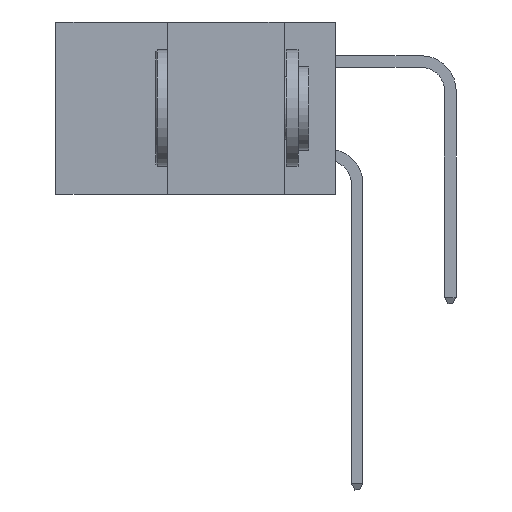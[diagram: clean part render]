
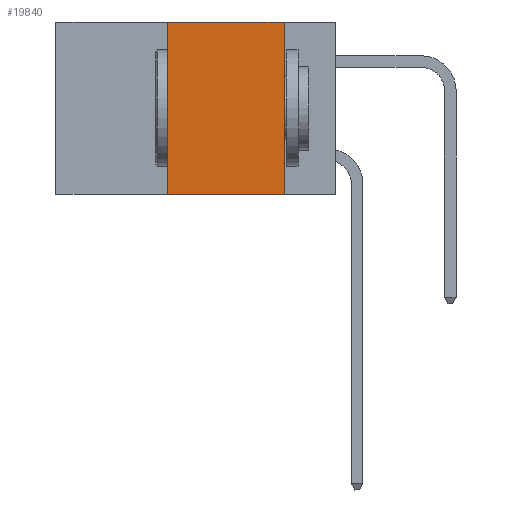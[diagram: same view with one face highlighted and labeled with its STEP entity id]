
A CAD part, left-side view. The second image highlights one B-rep face of the part: STEP entity #19840.
In plain terms, the highlighted planar face has unit normal (-1, 0, 0).
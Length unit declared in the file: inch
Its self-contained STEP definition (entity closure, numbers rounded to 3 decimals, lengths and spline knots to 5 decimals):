
#1787 = ORIENTED_EDGE ( 'NONE', *, *, #14523, .F. ) ;
#3164 = FACE_OUTER_BOUND ( 'NONE', #8803, .T. ) ;
#3603 = CARTESIAN_POINT ( 'NONE',  ( 0., 0.11, -0.37 ) ) ;
#3821 = VECTOR ( 'NONE', #36812, 39.37008 ) ;
#5599 = VECTOR ( 'NONE', #29644, 39.37008 ) ;
#8803 = EDGE_LOOP ( 'NONE', ( #12123, #22905, #1787, #17823 ) ) ;
#9039 = CARTESIAN_POINT ( 'NONE',  ( 0., 0.11, 0. ) ) ;
#9279 = VERTEX_POINT ( 'NONE', #35904 ) ;
#11865 = LINE ( 'NONE', #36172, #5599 ) ;
#12123 = ORIENTED_EDGE ( 'NONE', *, *, #18558, .F. ) ;
#14221 = CARTESIAN_POINT ( 'NONE',  ( 0., 0.36, 0. ) ) ;
#14462 = VERTEX_POINT ( 'NONE', #3603 ) ;
#14523 = EDGE_CURVE ( 'NONE', #9279, #37864, #28226, .T. ) ;
#14566 = VERTEX_POINT ( 'NONE', #9039 ) ;
#14584 = DIRECTION ( 'NONE',  ( 1., 0., 0. ) ) ;
#15663 = CARTESIAN_POINT ( 'NONE',  ( 0., 0.11, 0. ) ) ;
#17823 = ORIENTED_EDGE ( 'NONE', *, *, #21372, .T. ) ;
#17901 = DIRECTION ( 'NONE',  ( 0., 0., -1. ) ) ;
#18227 = DIRECTION ( 'NONE',  ( 0., 0., 1. ) ) ;
#18287 = VECTOR ( 'NONE', #18227, 39.37008 ) ;
#18558 = EDGE_CURVE ( 'NONE', #14566, #14462, #40916, .T. ) ;
#18963 = EDGE_CURVE ( 'NONE', #37864, #14566, #29916, .T. ) ;
#19840 = ADVANCED_FACE ( 'NONE', ( #3164 ), #24498, .F. ) ;
#21372 = EDGE_CURVE ( 'NONE', #9279, #14462, #11865, .T. ) ;
#22905 = ORIENTED_EDGE ( 'NONE', *, *, #18963, .F. ) ;
#24498 = PLANE ( 'NONE',  #36258 ) ;
#25441 = DIRECTION ( 'NONE',  ( 0., 0., -1. ) ) ;
#28226 = LINE ( 'NONE', #34012, #18287 ) ;
#29644 = DIRECTION ( 'NONE',  ( 0., -1., 0. ) ) ;
#29916 = LINE ( 'NONE', #29990, #3821 ) ;
#29990 = CARTESIAN_POINT ( 'NONE',  ( 0., 0.6, 0. ) ) ;
#34012 = CARTESIAN_POINT ( 'NONE',  ( 0., 0.36, 0. ) ) ;
#34552 = CARTESIAN_POINT ( 'NONE',  ( 0., 0.6, 0. ) ) ;
#35904 = CARTESIAN_POINT ( 'NONE',  ( 0., 0.36, -0.37 ) ) ;
#36172 = CARTESIAN_POINT ( 'NONE',  ( 0., 0.6, -0.37 ) ) ;
#36258 = AXIS2_PLACEMENT_3D ( 'NONE', #34552, #14584, #17901 ) ;
#36812 = DIRECTION ( 'NONE',  ( 0., -1., 0. ) ) ;
#37864 = VERTEX_POINT ( 'NONE', #14221 ) ;
#39878 = VECTOR ( 'NONE', #25441, 39.37008 ) ;
#40916 = LINE ( 'NONE', #15663, #39878 ) ;
